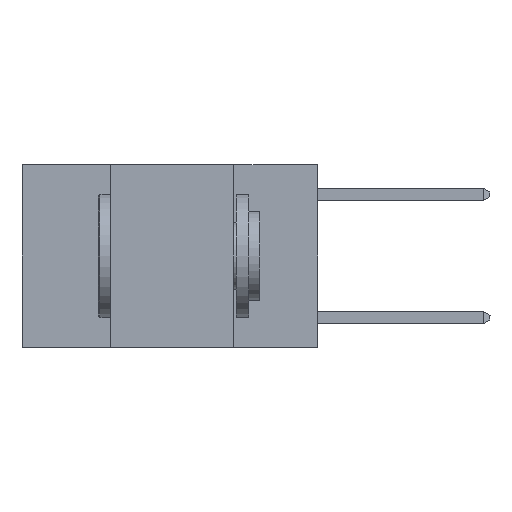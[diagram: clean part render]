
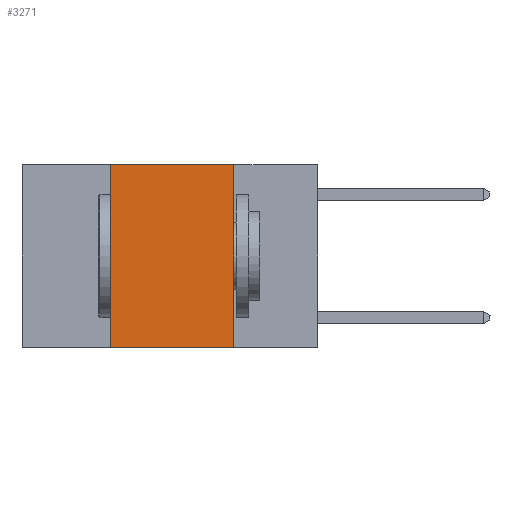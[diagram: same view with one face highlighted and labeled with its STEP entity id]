
A CAD part, left-side view. The second image highlights one B-rep face of the part: STEP entity #3271.
In plain terms, the highlighted planar face has unit normal (-1, 0, 0).
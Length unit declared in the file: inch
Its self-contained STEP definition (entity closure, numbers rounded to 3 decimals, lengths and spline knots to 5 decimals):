
#151 = CARTESIAN_POINT ( 'NONE',  ( 0., 0.17, 0. ) ) ;
#182 = LINE ( 'NONE', #151, #4857 ) ;
#451 = FACE_OUTER_BOUND ( 'NONE', #8038, .T. ) ;
#601 = EDGE_CURVE ( 'NONE', #7572, #7500, #4642, .T. ) ;
#748 = LINE ( 'NONE', #2213, #8461 ) ;
#912 = AXIS2_PLACEMENT_3D ( 'NONE', #9292, #3508, #4336 ) ;
#920 = ORIENTED_EDGE ( 'NONE', *, *, #601, .F. ) ;
#1256 = PLANE ( 'NONE',  #912 ) ;
#2112 = LINE ( 'NONE', #4318, #4111 ) ;
#2213 = CARTESIAN_POINT ( 'NONE',  ( 0., 0.6, -0.37 ) ) ;
#2580 = EDGE_CURVE ( 'NONE', #8895, #7572, #2112, .T. ) ;
#2610 = EDGE_CURVE ( 'NONE', #7500, #5459, #182, .T. ) ;
#3033 = CARTESIAN_POINT ( 'NONE',  ( 0., 0.17, 0. ) ) ;
#3093 = DIRECTION ( 'NONE',  ( 0., 0., -1. ) ) ;
#3271 = ADVANCED_FACE ( 'NONE', ( #451 ), #1256, .F. ) ;
#3508 = DIRECTION ( 'NONE',  ( 1., 0., 0. ) ) ;
#4111 = VECTOR ( 'NONE', #7206, 39.37008 ) ;
#4318 = CARTESIAN_POINT ( 'NONE',  ( 0., 0.42, 0. ) ) ;
#4336 = DIRECTION ( 'NONE',  ( 0., 0., -1. ) ) ;
#4521 = CARTESIAN_POINT ( 'NONE',  ( 0., 0.42, 0. ) ) ;
#4642 = LINE ( 'NONE', #8250, #6964 ) ;
#4857 = VECTOR ( 'NONE', #3093, 39.37008 ) ;
#5207 = ORIENTED_EDGE ( 'NONE', *, *, #2610, .F. ) ;
#5348 = DIRECTION ( 'NONE',  ( 0., -1., 0. ) ) ;
#5459 = VERTEX_POINT ( 'NONE', #9063 ) ;
#6012 = EDGE_CURVE ( 'NONE', #8895, #5459, #748, .T. ) ;
#6713 = CARTESIAN_POINT ( 'NONE',  ( 0., 0.42, -0.37 ) ) ;
#6964 = VECTOR ( 'NONE', #5348, 39.37008 ) ;
#7193 = ORIENTED_EDGE ( 'NONE', *, *, #2580, .F. ) ;
#7206 = DIRECTION ( 'NONE',  ( 0., 0., 1. ) ) ;
#7285 = ORIENTED_EDGE ( 'NONE', *, *, #6012, .T. ) ;
#7500 = VERTEX_POINT ( 'NONE', #3033 ) ;
#7572 = VERTEX_POINT ( 'NONE', #4521 ) ;
#7843 = DIRECTION ( 'NONE',  ( 0., -1., 0. ) ) ;
#8038 = EDGE_LOOP ( 'NONE', ( #5207, #920, #7193, #7285 ) ) ;
#8250 = CARTESIAN_POINT ( 'NONE',  ( 0., 0.6, 0. ) ) ;
#8461 = VECTOR ( 'NONE', #7843, 39.37008 ) ;
#8895 = VERTEX_POINT ( 'NONE', #6713 ) ;
#9063 = CARTESIAN_POINT ( 'NONE',  ( 0., 0.17, -0.37 ) ) ;
#9292 = CARTESIAN_POINT ( 'NONE',  ( 0., 0.6, 0. ) ) ;
